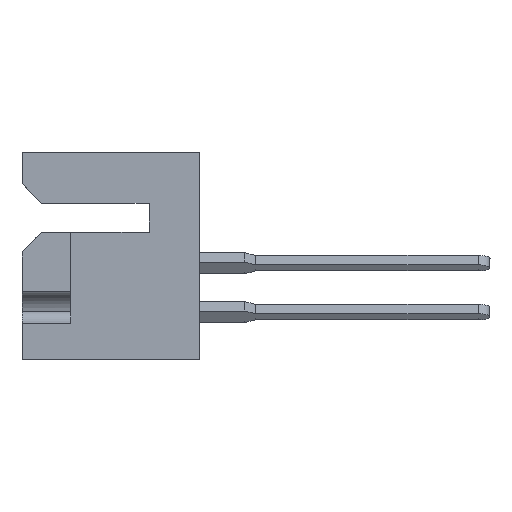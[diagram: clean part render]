
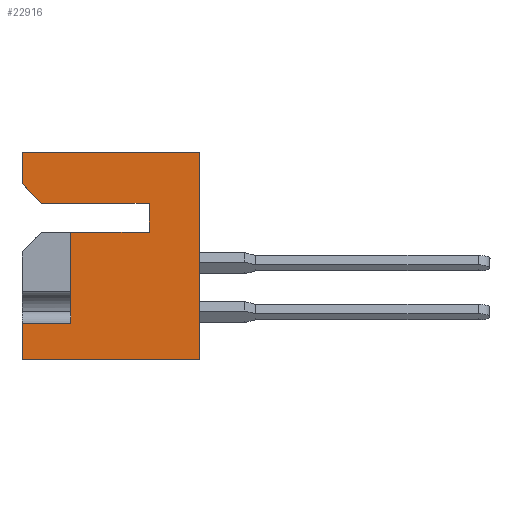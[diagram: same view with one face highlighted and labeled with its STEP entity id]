
A CAD part, left-side view. The second image highlights one B-rep face of the part: STEP entity #22916.
In plain terms, the highlighted planar face has unit normal (-1, 0, 0).
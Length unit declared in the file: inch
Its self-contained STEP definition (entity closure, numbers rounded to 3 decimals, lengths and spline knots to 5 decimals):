
#142 = DIRECTION ( 'NONE',  ( 0., 0., -1. ) ) ;
#156 = VERTEX_POINT ( 'NONE', #15923 ) ;
#285 = VECTOR ( 'NONE', #20568, 39.37008 ) ;
#607 = VECTOR ( 'NONE', #22329, 39.37008 ) ;
#817 = LINE ( 'NONE', #4128, #9687 ) ;
#979 = EDGE_CURVE ( 'NONE', #9673, #19714, #1021, .T. ) ;
#1021 = LINE ( 'NONE', #19504, #16810 ) ;
#1252 = VERTEX_POINT ( 'NONE', #20220 ) ;
#1638 = VERTEX_POINT ( 'NONE', #21303 ) ;
#1875 = CARTESIAN_POINT ( 'NONE',  ( 0., 0.453, 0. ) ) ;
#1895 = VECTOR ( 'NONE', #16881, 39.37008 ) ;
#2892 = CARTESIAN_POINT ( 'NONE',  ( 0., 0.453, -0.531 ) ) ;
#3339 = VECTOR ( 'NONE', #20155, 39.37008 ) ;
#4128 = CARTESIAN_POINT ( 'NONE',  ( 0., 0.453, 0. ) ) ;
#4212 = DIRECTION ( 'NONE',  ( 0., 0., 1. ) ) ;
#5446 = CARTESIAN_POINT ( 'NONE',  ( 0., 0.403, -0.131 ) ) ;
#5692 = VERTEX_POINT ( 'NONE', #25226 ) ;
#5878 = LINE ( 'NONE', #15859, #607 ) ;
#5883 = DIRECTION ( 'NONE',  ( 0., 1., 0. ) ) ;
#5964 = VERTEX_POINT ( 'NONE', #2892 ) ;
#6213 = VERTEX_POINT ( 'NONE', #1875 ) ;
#6295 = CARTESIAN_POINT ( 'NONE',  ( 0., 0.403, -0.131 ) ) ;
#6629 = LINE ( 'NONE', #21413, #8590 ) ;
#7009 = LINE ( 'NONE', #17513, #24420 ) ;
#7473 = LINE ( 'NONE', #14748, #1895 ) ;
#7495 = VERTEX_POINT ( 'NONE', #19175 ) ;
#7502 = DIRECTION ( 'NONE',  ( 0., 0., 1. ) ) ;
#7823 = VERTEX_POINT ( 'NONE', #12137 ) ;
#8590 = VECTOR ( 'NONE', #21238, 39.37008 ) ;
#8635 = CARTESIAN_POINT ( 'NONE',  ( 0., 0.128, -0.205 ) ) ;
#8674 = DIRECTION ( 'NONE',  ( 1., 0., 0. ) ) ;
#9566 = ORIENTED_EDGE ( 'NONE', *, *, #22332, .F. ) ;
#9577 = CARTESIAN_POINT ( 'NONE',  ( 0., 0.328, -0.205 ) ) ;
#9673 = VERTEX_POINT ( 'NONE', #8635 ) ;
#9687 = VECTOR ( 'NONE', #4212, 39.37008 ) ;
#10066 = CARTESIAN_POINT ( 'NONE',  ( 0., 0.128, -0.205 ) ) ;
#10566 = AXIS2_PLACEMENT_3D ( 'NONE', #14532, #8674, #142 ) ;
#10760 = VECTOR ( 'NONE', #17290, 39.37008 ) ;
#10870 = EDGE_CURVE ( 'NONE', #5692, #1252, #7009, .T. ) ;
#11105 = DIRECTION ( 'NONE',  ( 0., 0., 1. ) ) ;
#11330 = ORIENTED_EDGE ( 'NONE', *, *, #22864, .F. ) ;
#11376 = EDGE_CURVE ( 'NONE', #9673, #156, #22424, .T. ) ;
#12137 = CARTESIAN_POINT ( 'NONE',  ( 0., 0.453, -0.437 ) ) ;
#12167 = ORIENTED_EDGE ( 'NONE', *, *, #15669, .F. ) ;
#13169 = DIRECTION ( 'NONE',  ( 0., 0., 1. ) ) ;
#13375 = EDGE_LOOP ( 'NONE', ( #23424, #9566, #20576, #13485, #17968, #17622, #23781, #11330, #14832, #18254, #12167 ) ) ;
#13485 = ORIENTED_EDGE ( 'NONE', *, *, #10870, .T. ) ;
#14489 = LINE ( 'NONE', #5446, #3339 ) ;
#14532 = CARTESIAN_POINT ( 'NONE',  ( 0., 0.453, 0. ) ) ;
#14748 = CARTESIAN_POINT ( 'NONE',  ( 0., 0.453, 0. ) ) ;
#14832 = ORIENTED_EDGE ( 'NONE', *, *, #979, .F. ) ;
#15145 = CARTESIAN_POINT ( 'NONE',  ( 0., 0.453, -0.531 ) ) ;
#15669 = EDGE_CURVE ( 'NONE', #1638, #156, #24805, .T. ) ;
#15859 = CARTESIAN_POINT ( 'NONE',  ( 0., 0.328, -0.437 ) ) ;
#15923 = CARTESIAN_POINT ( 'NONE',  ( 0., 0.328, -0.205 ) ) ;
#16810 = VECTOR ( 'NONE', #11105, 39.37008 ) ;
#16881 = DIRECTION ( 'NONE',  ( 0., 0., 1. ) ) ;
#17290 = DIRECTION ( 'NONE',  ( 0., -1., 0. ) ) ;
#17513 = CARTESIAN_POINT ( 'NONE',  ( 0., 0., 0. ) ) ;
#17622 = ORIENTED_EDGE ( 'NONE', *, *, #26066, .F. ) ;
#17968 = ORIENTED_EDGE ( 'NONE', *, *, #18703, .F. ) ;
#18254 = ORIENTED_EDGE ( 'NONE', *, *, #11376, .T. ) ;
#18326 = EDGE_CURVE ( 'NONE', #7495, #25360, #14489, .T. ) ;
#18342 = LINE ( 'NONE', #15145, #10760 ) ;
#18373 = LINE ( 'NONE', #27057, #285 ) ;
#18703 = EDGE_CURVE ( 'NONE', #6213, #1252, #6629, .T. ) ;
#19175 = CARTESIAN_POINT ( 'NONE',  ( 0., 0.453, -0.081 ) ) ;
#19504 = CARTESIAN_POINT ( 'NONE',  ( 0., 0.128, -0.131 ) ) ;
#19714 = VERTEX_POINT ( 'NONE', #20180 ) ;
#20155 = DIRECTION ( 'NONE',  ( 0., -0.707, -0.707 ) ) ;
#20180 = CARTESIAN_POINT ( 'NONE',  ( 0., 0.128, -0.131 ) ) ;
#20220 = CARTESIAN_POINT ( 'NONE',  ( 0., 0., 0. ) ) ;
#20310 = EDGE_CURVE ( 'NONE', #1638, #7823, #5878, .T. ) ;
#20568 = DIRECTION ( 'NONE',  ( 0., 1., 0. ) ) ;
#20576 = ORIENTED_EDGE ( 'NONE', *, *, #25470, .T. ) ;
#20920 = PLANE ( 'NONE',  #10566 ) ;
#21179 = VECTOR ( 'NONE', #7502, 39.37008 ) ;
#21238 = DIRECTION ( 'NONE',  ( 0., -1., 0. ) ) ;
#21286 = FACE_OUTER_BOUND ( 'NONE', #13375, .T. ) ;
#21303 = CARTESIAN_POINT ( 'NONE',  ( 0., 0.328, -0.437 ) ) ;
#21413 = CARTESIAN_POINT ( 'NONE',  ( 0., 0.453, 0. ) ) ;
#22329 = DIRECTION ( 'NONE',  ( 0., 1., 0. ) ) ;
#22332 = EDGE_CURVE ( 'NONE', #5964, #7823, #817, .T. ) ;
#22424 = LINE ( 'NONE', #10066, #23753 ) ;
#22864 = EDGE_CURVE ( 'NONE', #19714, #25360, #18373, .T. ) ;
#22916 = ADVANCED_FACE ( 'NONE', ( #21286 ), #20920, .F. ) ;
#23424 = ORIENTED_EDGE ( 'NONE', *, *, #20310, .T. ) ;
#23753 = VECTOR ( 'NONE', #5883, 39.37008 ) ;
#23781 = ORIENTED_EDGE ( 'NONE', *, *, #18326, .T. ) ;
#24420 = VECTOR ( 'NONE', #13169, 39.37008 ) ;
#24805 = LINE ( 'NONE', #9577, #21179 ) ;
#25226 = CARTESIAN_POINT ( 'NONE',  ( 0., 0., -0.531 ) ) ;
#25360 = VERTEX_POINT ( 'NONE', #6295 ) ;
#25470 = EDGE_CURVE ( 'NONE', #5964, #5692, #18342, .T. ) ;
#26066 = EDGE_CURVE ( 'NONE', #7495, #6213, #7473, .T. ) ;
#27057 = CARTESIAN_POINT ( 'NONE',  ( 0., 0.128, -0.131 ) ) ;
